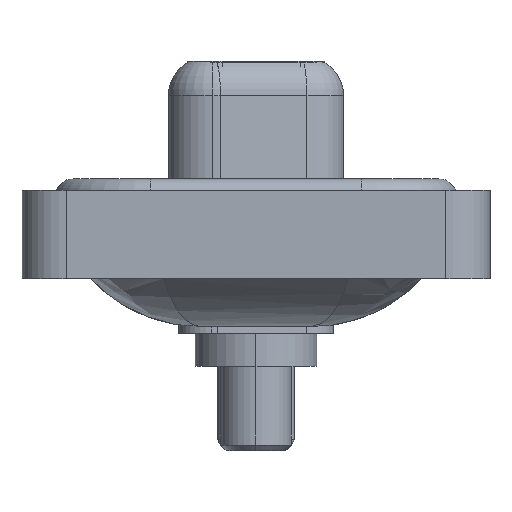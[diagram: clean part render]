
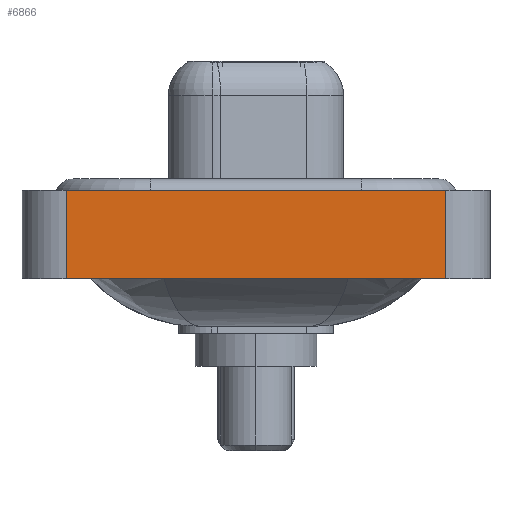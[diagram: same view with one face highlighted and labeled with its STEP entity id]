
A CAD part, left-side view. The second image highlights one B-rep face of the part: STEP entity #6866.
In plain terms, the highlighted planar face has unit normal (-1, 0, 0).
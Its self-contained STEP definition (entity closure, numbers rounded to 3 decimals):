
#589 = FACE_OUTER_BOUND ( 'NONE', #12704, .T. ) ;
#690 = LINE ( 'NONE', #8520, #23454 ) ;
#2030 = CARTESIAN_POINT ( 'NONE',  ( -7.35, 8.55, -3.6 ) ) ;
#2466 = CARTESIAN_POINT ( 'NONE',  ( -7.35, -8.55, 0.4 ) ) ;
#2831 = VECTOR ( 'NONE', #21388, 1000. ) ;
#3002 = DIRECTION ( 'NONE',  ( 0., -1., 0. ) ) ;
#3832 = DIRECTION ( 'NONE',  ( -1., 0., 0. ) ) ;
#6866 = ADVANCED_FACE ( 'NONE', ( #589 ), #22968, .T. ) ;
#7846 = CARTESIAN_POINT ( 'NONE',  ( -7.35, -8.55, -3.6 ) ) ;
#7859 = CARTESIAN_POINT ( 'NONE',  ( -7.35, -8.55, -3.6 ) ) ;
#7962 = VERTEX_POINT ( 'NONE', #2466 ) ;
#8219 = VERTEX_POINT ( 'NONE', #12786 ) ;
#8520 = CARTESIAN_POINT ( 'NONE',  ( -7.35, -8.55, 0.4 ) ) ;
#8589 = EDGE_CURVE ( 'NONE', #8219, #7962, #690, .T. ) ;
#8769 = DIRECTION ( 'NONE',  ( 0., -1., 0. ) ) ;
#8951 = ORIENTED_EDGE ( 'NONE', *, *, #10205, .T. ) ;
#10205 = EDGE_CURVE ( 'NONE', #17605, #7962, #21264, .T. ) ;
#10651 = VECTOR ( 'NONE', #3002, 1000. ) ;
#10756 = CARTESIAN_POINT ( 'NONE',  ( -7.35, 8.55, -3.6 ) ) ;
#11421 = DIRECTION ( 'NONE',  ( 0., 0., 1. ) ) ;
#11867 = EDGE_CURVE ( 'NONE', #21736, #17605, #18305, .T. ) ;
#12704 = EDGE_LOOP ( 'NONE', ( #8951, #18077, #13148, #17619 ) ) ;
#12786 = CARTESIAN_POINT ( 'NONE',  ( -7.35, 8.55, 0.4 ) ) ;
#13148 = ORIENTED_EDGE ( 'NONE', *, *, #21213, .F. ) ;
#15121 = DIRECTION ( 'NONE',  ( 0., 0., 1. ) ) ;
#15315 = VECTOR ( 'NONE', #15121, 1000. ) ;
#15747 = CARTESIAN_POINT ( 'NONE',  ( -7.35, -8.55, -3.6 ) ) ;
#16056 = CARTESIAN_POINT ( 'NONE',  ( -7.35, -8.55, -3.6 ) ) ;
#17605 = VERTEX_POINT ( 'NONE', #7859 ) ;
#17619 = ORIENTED_EDGE ( 'NONE', *, *, #11867, .T. ) ;
#18077 = ORIENTED_EDGE ( 'NONE', *, *, #8589, .F. ) ;
#18305 = LINE ( 'NONE', #16056, #10651 ) ;
#18608 = AXIS2_PLACEMENT_3D ( 'NONE', #15747, #3832, #11421 ) ;
#20445 = LINE ( 'NONE', #10756, #15315 ) ;
#21213 = EDGE_CURVE ( 'NONE', #21736, #8219, #20445, .T. ) ;
#21264 = LINE ( 'NONE', #7846, #2831 ) ;
#21388 = DIRECTION ( 'NONE',  ( 0., 0., 1. ) ) ;
#21736 = VERTEX_POINT ( 'NONE', #2030 ) ;
#22968 = PLANE ( 'NONE',  #18608 ) ;
#23454 = VECTOR ( 'NONE', #8769, 1000. ) ;
